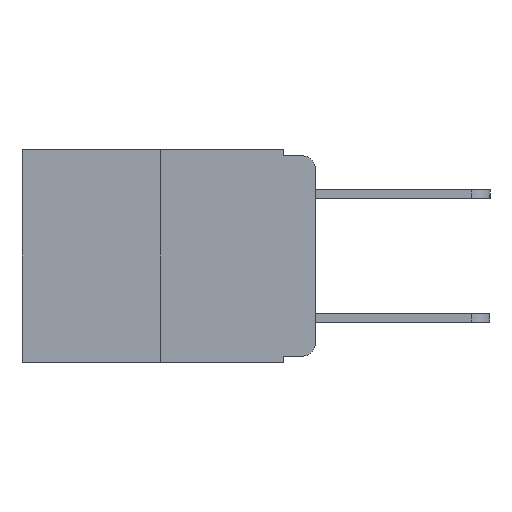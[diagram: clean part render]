
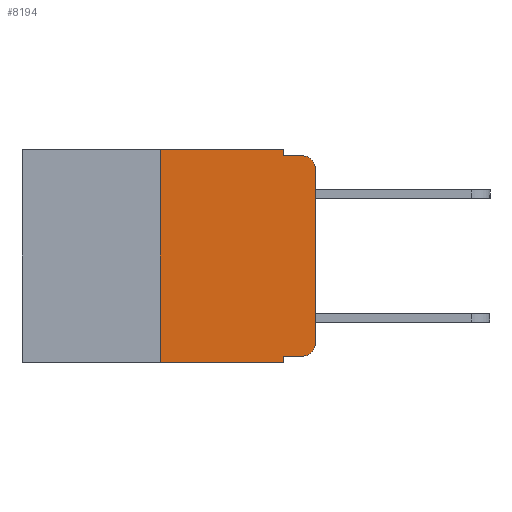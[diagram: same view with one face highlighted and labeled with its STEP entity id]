
A CAD part, left-side view. The second image highlights one B-rep face of the part: STEP entity #8194.
In plain terms, the highlighted planar face has unit normal (-1, 0, 0).
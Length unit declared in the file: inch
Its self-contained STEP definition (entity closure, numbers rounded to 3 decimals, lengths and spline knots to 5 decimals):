
#155 = VERTEX_POINT ( 'NONE', #8497 ) ;
#210 = VECTOR ( 'NONE', #9699, 39.37008 ) ;
#482 = DIRECTION ( 'NONE',  ( 0., 0., -1. ) ) ;
#528 = DIRECTION ( 'NONE',  ( 1., 0., 0. ) ) ;
#649 = AXIS2_PLACEMENT_3D ( 'NONE', #5990, #5629, #5890 ) ;
#914 = EDGE_CURVE ( 'NONE', #4412, #155, #8910, .T. ) ;
#1020 = ORIENTED_EDGE ( 'NONE', *, *, #914, .F. ) ;
#1120 = CARTESIAN_POINT ( 'NONE',  ( 0., 0., -0.313 ) ) ;
#1240 = PLANE ( 'NONE',  #6620 ) ;
#1334 = LINE ( 'NONE', #5640, #5374 ) ;
#1482 = LINE ( 'NONE', #3288, #5494 ) ;
#1500 = CARTESIAN_POINT ( 'NONE',  ( 0., 0.473, 0. ) ) ;
#1766 = EDGE_LOOP ( 'NONE', ( #6339, #7953, #2669, #2693, #1020, #4525, #4431, #4374, #4288, #3855 ) ) ;
#1975 = CARTESIAN_POINT ( 'NONE',  ( 0., 0.051, 0. ) ) ;
#2162 = VERTEX_POINT ( 'NONE', #7749 ) ;
#2585 = EDGE_CURVE ( 'NONE', #6569, #3464, #2860, .T. ) ;
#2589 = CARTESIAN_POINT ( 'NONE',  ( 0., 0.25, -0.343 ) ) ;
#2669 = ORIENTED_EDGE ( 'NONE', *, *, #4084, .F. ) ;
#2693 = ORIENTED_EDGE ( 'NONE', *, *, #4134, .F. ) ;
#2860 = LINE ( 'NONE', #7107, #8626 ) ;
#2955 = LINE ( 'NONE', #3515, #8954 ) ;
#3288 = CARTESIAN_POINT ( 'NONE',  ( 0., 0.25, 0. ) ) ;
#3358 = DIRECTION ( 'NONE',  ( 0., -1., 0. ) ) ;
#3454 = VERTEX_POINT ( 'NONE', #6130 ) ;
#3464 = VERTEX_POINT ( 'NONE', #6017 ) ;
#3515 = CARTESIAN_POINT ( 'NONE',  ( 0., 0.051, 0. ) ) ;
#3525 = DIRECTION ( 'NONE',  ( 0., 0., -1. ) ) ;
#3549 = CARTESIAN_POINT ( 'NONE',  ( 0., 0.051, -0.333 ) ) ;
#3607 = CIRCLE ( 'NONE', #649, 0.02 ) ;
#3855 = ORIENTED_EDGE ( 'NONE', *, *, #4450, .T. ) ;
#3992 = DIRECTION ( 'NONE',  ( 0., -1., 0. ) ) ;
#4050 = EDGE_CURVE ( 'NONE', #7288, #2162, #7718, .T. ) ;
#4072 = AXIS2_PLACEMENT_3D ( 'NONE', #8826, #4465, #4507 ) ;
#4083 = EDGE_CURVE ( 'NONE', #2162, #3454, #3607, .T. ) ;
#4084 = EDGE_CURVE ( 'NONE', #5697, #3454, #1334, .T. ) ;
#4134 = EDGE_CURVE ( 'NONE', #155, #5697, #5155, .T. ) ;
#4278 = EDGE_CURVE ( 'NONE', #6569, #4412, #1482, .T. ) ;
#4288 = ORIENTED_EDGE ( 'NONE', *, *, #4436, .T. ) ;
#4374 = ORIENTED_EDGE ( 'NONE', *, *, #4387, .F. ) ;
#4387 = EDGE_CURVE ( 'NONE', #8469, #3464, #2955, .T. ) ;
#4412 = VERTEX_POINT ( 'NONE', #5818 ) ;
#4431 = ORIENTED_EDGE ( 'NONE', *, *, #2585, .T. ) ;
#4436 = EDGE_CURVE ( 'NONE', #8469, #5938, #6804, .T. ) ;
#4450 = EDGE_CURVE ( 'NONE', #5938, #7288, #6552, .T. ) ;
#4465 = DIRECTION ( 'NONE',  ( -1., 0., 0. ) ) ;
#4507 = DIRECTION ( 'NONE',  ( 0., 0., -1. ) ) ;
#4525 = ORIENTED_EDGE ( 'NONE', *, *, #4278, .F. ) ;
#4813 = VECTOR ( 'NONE', #3358, 39.37008 ) ;
#4989 = CARTESIAN_POINT ( 'NONE',  ( 0., 0., 0. ) ) ;
#5155 = LINE ( 'NONE', #1975, #210 ) ;
#5374 = VECTOR ( 'NONE', #5672, 39.37008 ) ;
#5494 = VECTOR ( 'NONE', #6349, 39.37008 ) ;
#5611 = DIRECTION ( 'NONE',  ( 0., 0., 1. ) ) ;
#5628 = VECTOR ( 'NONE', #5611, 39.37008 ) ;
#5629 = DIRECTION ( 'NONE',  ( -1., 0., 0. ) ) ;
#5640 = CARTESIAN_POINT ( 'NONE',  ( 0., 0.051, -0.01 ) ) ;
#5672 = DIRECTION ( 'NONE',  ( 0., -1., 0. ) ) ;
#5697 = VERTEX_POINT ( 'NONE', #8822 ) ;
#5818 = CARTESIAN_POINT ( 'NONE',  ( 0., 0.25, 0. ) ) ;
#5890 = DIRECTION ( 'NONE',  ( 0., 0., -1. ) ) ;
#5938 = VERTEX_POINT ( 'NONE', #6397 ) ;
#5990 = CARTESIAN_POINT ( 'NONE',  ( 0., 0.02, -0.03 ) ) ;
#6017 = CARTESIAN_POINT ( 'NONE',  ( 0., 0.051, -0.343 ) ) ;
#6130 = CARTESIAN_POINT ( 'NONE',  ( 0., 0.02, -0.01 ) ) ;
#6339 = ORIENTED_EDGE ( 'NONE', *, *, #4050, .T. ) ;
#6349 = DIRECTION ( 'NONE',  ( 0., 0., 1. ) ) ;
#6397 = CARTESIAN_POINT ( 'NONE',  ( 0., 0.02, -0.333 ) ) ;
#6552 = CIRCLE ( 'NONE', #4072, 0.02 ) ;
#6569 = VERTEX_POINT ( 'NONE', #2589 ) ;
#6620 = AXIS2_PLACEMENT_3D ( 'NONE', #1500, #528, #482 ) ;
#6804 = LINE ( 'NONE', #3549, #4813 ) ;
#6965 = DIRECTION ( 'NONE',  ( 0., -1., 0. ) ) ;
#7107 = CARTESIAN_POINT ( 'NONE',  ( 0., 0.473, -0.343 ) ) ;
#7288 = VERTEX_POINT ( 'NONE', #1120 ) ;
#7718 = LINE ( 'NONE', #4989, #5628 ) ;
#7749 = CARTESIAN_POINT ( 'NONE',  ( 0., 0., -0.03 ) ) ;
#7953 = ORIENTED_EDGE ( 'NONE', *, *, #4083, .T. ) ;
#8194 = ADVANCED_FACE ( 'NONE', ( #9564 ), #1240, .F. ) ;
#8469 = VERTEX_POINT ( 'NONE', #8617 ) ;
#8497 = CARTESIAN_POINT ( 'NONE',  ( 0., 0.051, 0. ) ) ;
#8617 = CARTESIAN_POINT ( 'NONE',  ( 0., 0.051, -0.333 ) ) ;
#8626 = VECTOR ( 'NONE', #6965, 39.37008 ) ;
#8656 = VECTOR ( 'NONE', #3992, 39.37008 ) ;
#8822 = CARTESIAN_POINT ( 'NONE',  ( 0., 0.051, -0.01 ) ) ;
#8826 = CARTESIAN_POINT ( 'NONE',  ( 0., 0.02, -0.313 ) ) ;
#8910 = LINE ( 'NONE', #9088, #8656 ) ;
#8954 = VECTOR ( 'NONE', #3525, 39.37008 ) ;
#9088 = CARTESIAN_POINT ( 'NONE',  ( 0., 0.473, 0. ) ) ;
#9564 = FACE_OUTER_BOUND ( 'NONE', #1766, .T. ) ;
#9699 = DIRECTION ( 'NONE',  ( 0., 0., -1. ) ) ;
